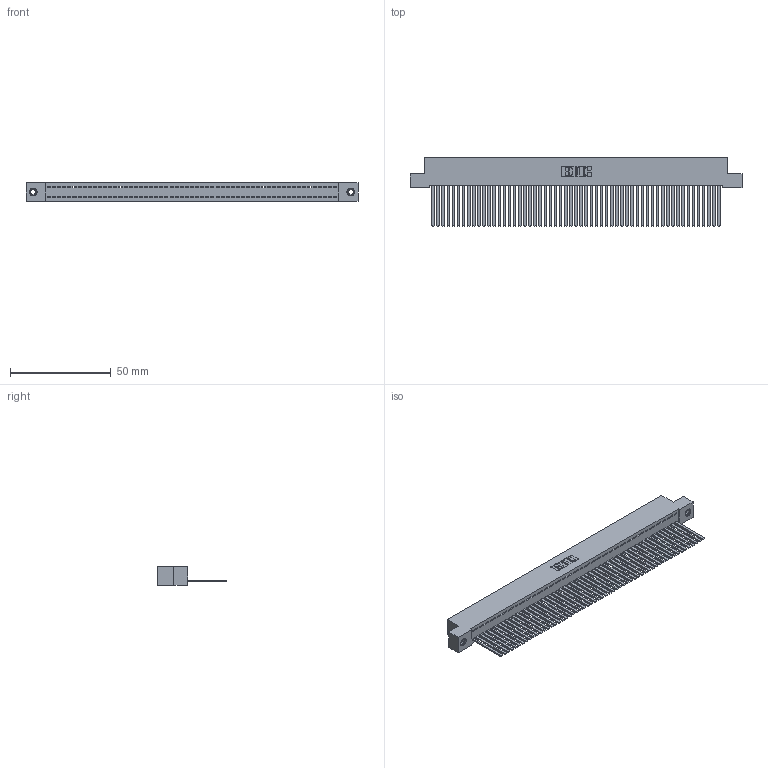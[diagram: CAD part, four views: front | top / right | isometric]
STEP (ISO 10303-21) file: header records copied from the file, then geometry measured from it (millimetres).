
FILE_DESCRIPTION (( 'STEP AP203' ), '1' );
FILE_NAME ('392-057-544-108.STEP', '2018-08-17T15:31:22', ( '' ), ( '' ), 'SwSTEP 2.0', 'SolidWorks 2016', '' );
FILE_SCHEMA (( 'CONFIG_CONTROL_DESIGN' ));
Length unit declared in the file: inch
Products named in the file (4): 342 Part_TI; 345-292-001_345-293-144; 345-250-001_345-250-003-102; 392-057-544-108
Assembly tree (60 placements, depth 2):
  392-057-544-108
    342 Part_TI
    345-292-001_345-293-144  x57
    345-250-001_345-250-003-102  x2
Bounding box: 165.1 x 34.3 x 9.4 mm (x, y, z)
Volume: 15185.7 mm3; surface area: 24476.2 mm2
Topology: 60 solids, 60 shells, 3134 faces, 9441 edges, 6210 vertices
Faces by surface type: plane 2264, cylinder 854, cone 12, torus 4
Entity records: 33776 total; most frequent: CARTESIAN_POINT 5804, ORIENTED_EDGE 5790, DIRECTION 4895, EDGE_CURVE 2895, LINE 2751, VECTOR 2751, VERTEX_POINT 1924, AXIS2_PLACEMENT_3D 1072
